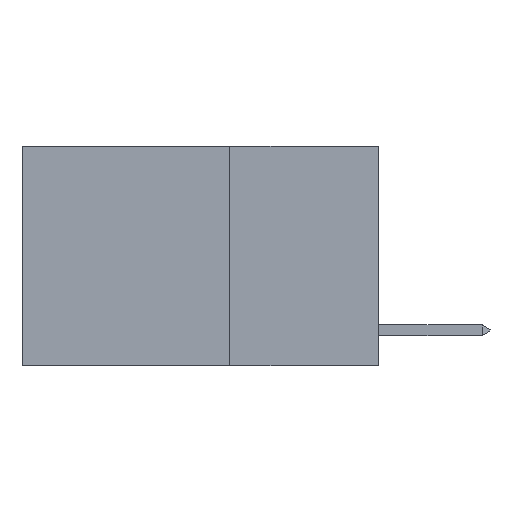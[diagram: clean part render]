
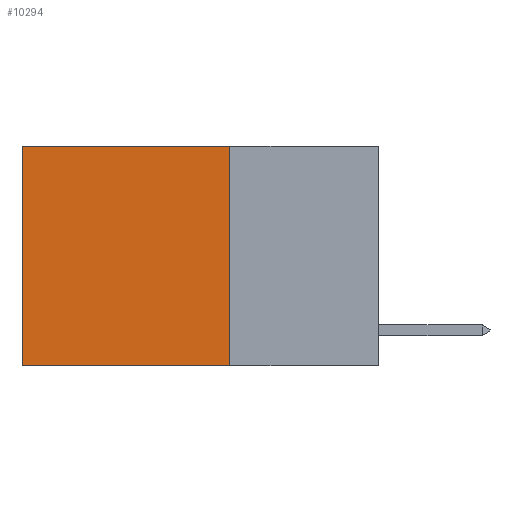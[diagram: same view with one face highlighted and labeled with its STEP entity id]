
A CAD part, left-side view. The second image highlights one B-rep face of the part: STEP entity #10294.
In plain terms, the highlighted planar face has unit normal (-1, 0, 0).
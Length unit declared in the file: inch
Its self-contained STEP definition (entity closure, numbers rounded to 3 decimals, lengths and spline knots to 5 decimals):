
#17 = PLANE ( 'NONE',  #7041 ) ;
#327 = DIRECTION ( 'NONE',  ( 0., 0., -1. ) ) ;
#926 = LINE ( 'NONE', #17670, #6901 ) ;
#1247 = LINE ( 'NONE', #16884, #10188 ) ;
#3920 = VERTEX_POINT ( 'NONE', #15875 ) ;
#4378 = DIRECTION ( 'NONE',  ( 0., 1., 0. ) ) ;
#4517 = EDGE_CURVE ( 'NONE', #7268, #3920, #1247, .T. ) ;
#4565 = VERTEX_POINT ( 'NONE', #5887 ) ;
#4646 = DIRECTION ( 'NONE',  ( 0., 0., -1. ) ) ;
#5425 = VECTOR ( 'NONE', #4646, 39.37008 ) ;
#5887 = CARTESIAN_POINT ( 'NONE',  ( 0.2625, 0.6, -0.37 ) ) ;
#6215 = DIRECTION ( 'NONE',  ( 0., 0., -1. ) ) ;
#6901 = VECTOR ( 'NONE', #18969, 39.37008 ) ;
#7041 = AXIS2_PLACEMENT_3D ( 'NONE', #7984, #15192, #327 ) ;
#7268 = VERTEX_POINT ( 'NONE', #9804 ) ;
#7653 = LINE ( 'NONE', #15166, #5425 ) ;
#7685 = FACE_OUTER_BOUND ( 'NONE', #11807, .T. ) ;
#7984 = CARTESIAN_POINT ( 'NONE',  ( 0.2625, 0.25, 0. ) ) ;
#8050 = ORIENTED_EDGE ( 'NONE', *, *, #4517, .T. ) ;
#8970 = ORIENTED_EDGE ( 'NONE', *, *, #16928, .T. ) ;
#9804 = CARTESIAN_POINT ( 'NONE',  ( 0.2625, 0.25, 0. ) ) ;
#10188 = VECTOR ( 'NONE', #4378, 39.37008 ) ;
#10294 = ADVANCED_FACE ( 'NONE', ( #7685 ), #17, .F. ) ;
#10604 = EDGE_CURVE ( 'NONE', #7268, #13330, #7653, .T. ) ;
#11623 = VECTOR ( 'NONE', #6215, 39.37008 ) ;
#11807 = EDGE_LOOP ( 'NONE', ( #8970, #15481, #18990, #8050 ) ) ;
#13330 = VERTEX_POINT ( 'NONE', #15038 ) ;
#15038 = CARTESIAN_POINT ( 'NONE',  ( 0.2625, 0.25, -0.37 ) ) ;
#15166 = CARTESIAN_POINT ( 'NONE',  ( 0.2625, 0.25, 0. ) ) ;
#15192 = DIRECTION ( 'NONE',  ( 1., 0., 0. ) ) ;
#15481 = ORIENTED_EDGE ( 'NONE', *, *, #18062, .F. ) ;
#15875 = CARTESIAN_POINT ( 'NONE',  ( 0.2625, 0.6, 0. ) ) ;
#16884 = CARTESIAN_POINT ( 'NONE',  ( 0.2625, 0.25, 0. ) ) ;
#16926 = CARTESIAN_POINT ( 'NONE',  ( 0.2625, 0.6, 0. ) ) ;
#16928 = EDGE_CURVE ( 'NONE', #3920, #4565, #19610, .T. ) ;
#17670 = CARTESIAN_POINT ( 'NONE',  ( 0.2625, 0.25, -0.37 ) ) ;
#18062 = EDGE_CURVE ( 'NONE', #13330, #4565, #926, .T. ) ;
#18969 = DIRECTION ( 'NONE',  ( 0., 1., 0. ) ) ;
#18990 = ORIENTED_EDGE ( 'NONE', *, *, #10604, .F. ) ;
#19610 = LINE ( 'NONE', #16926, #11623 ) ;
